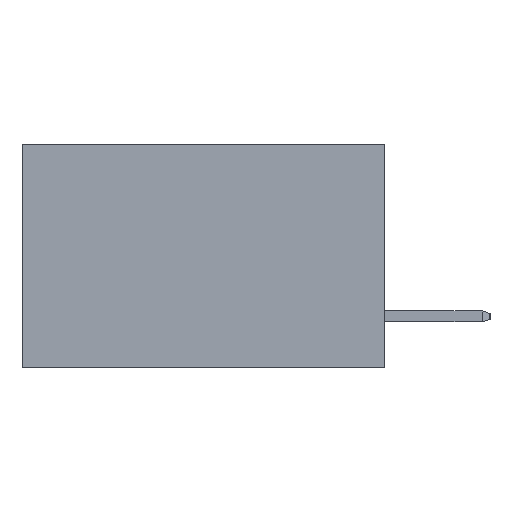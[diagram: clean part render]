
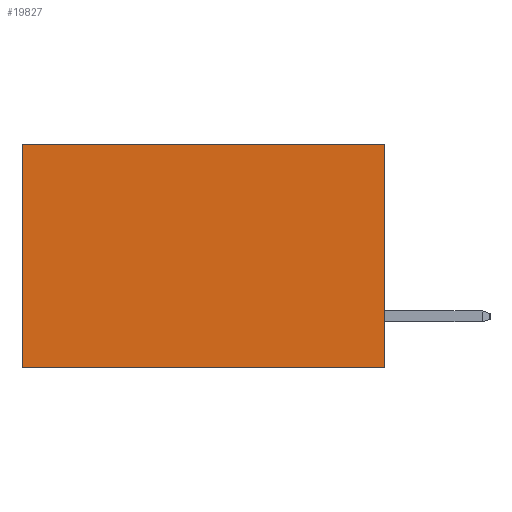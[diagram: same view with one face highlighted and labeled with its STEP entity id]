
A CAD part, left-side view. The second image highlights one B-rep face of the part: STEP entity #19827.
In plain terms, the highlighted planar face has unit normal (-1, 0, 0).
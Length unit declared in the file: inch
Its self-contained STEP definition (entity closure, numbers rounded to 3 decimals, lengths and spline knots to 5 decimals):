
#311 = DIRECTION ( 'NONE',  ( 0., 1., 0. ) ) ;
#355 = LINE ( 'NONE', #21070, #23672 ) ;
#1410 = DIRECTION ( 'NONE',  ( 0., 0., -1. ) ) ;
#2884 = CARTESIAN_POINT ( 'NONE',  ( 0.298, 0.6, 0. ) ) ;
#3209 = FACE_OUTER_BOUND ( 'NONE', #24162, .T. ) ;
#4001 = VERTEX_POINT ( 'NONE', #15580 ) ;
#4132 = ORIENTED_EDGE ( 'NONE', *, *, #22216, .F. ) ;
#4339 = LINE ( 'NONE', #30068, #28302 ) ;
#4352 = ORIENTED_EDGE ( 'NONE', *, *, #30662, .T. ) ;
#6212 = DIRECTION ( 'NONE',  ( 1., 0., 0. ) ) ;
#6879 = LINE ( 'NONE', #30172, #25953 ) ;
#8202 = CARTESIAN_POINT ( 'NONE',  ( 0.298, 0.6, -0.37 ) ) ;
#13429 = VECTOR ( 'NONE', #311, 39.37008 ) ;
#13577 = DIRECTION ( 'NONE',  ( 0., 0., -1. ) ) ;
#13687 = AXIS2_PLACEMENT_3D ( 'NONE', #20580, #6212, #22971 ) ;
#13732 = ORIENTED_EDGE ( 'NONE', *, *, #15930, .T. ) ;
#14002 = DIRECTION ( 'NONE',  ( 0., 1., 0. ) ) ;
#15580 = CARTESIAN_POINT ( 'NONE',  ( 0.298, 0., 0. ) ) ;
#15930 = EDGE_CURVE ( 'NONE', #25915, #20341, #6879, .T. ) ;
#17226 = VERTEX_POINT ( 'NONE', #24943 ) ;
#19485 = CARTESIAN_POINT ( 'NONE',  ( 0.298, 0., 0. ) ) ;
#19759 = LINE ( 'NONE', #19485, #13429 ) ;
#19827 = ADVANCED_FACE ( 'NONE', ( #3209 ), #25247, .F. ) ;
#20341 = VERTEX_POINT ( 'NONE', #8202 ) ;
#20580 = CARTESIAN_POINT ( 'NONE',  ( 0.298, 0., 0. ) ) ;
#21070 = CARTESIAN_POINT ( 'NONE',  ( 0.298, 0., -0.37 ) ) ;
#21430 = ORIENTED_EDGE ( 'NONE', *, *, #27681, .F. ) ;
#22216 = EDGE_CURVE ( 'NONE', #4001, #17226, #4339, .T. ) ;
#22971 = DIRECTION ( 'NONE',  ( 0., 0., -1. ) ) ;
#23672 = VECTOR ( 'NONE', #14002, 39.37008 ) ;
#24162 = EDGE_LOOP ( 'NONE', ( #13732, #21430, #4132, #4352 ) ) ;
#24943 = CARTESIAN_POINT ( 'NONE',  ( 0.298, 0., -0.37 ) ) ;
#25247 = PLANE ( 'NONE',  #13687 ) ;
#25915 = VERTEX_POINT ( 'NONE', #2884 ) ;
#25953 = VECTOR ( 'NONE', #13577, 39.37008 ) ;
#27681 = EDGE_CURVE ( 'NONE', #17226, #20341, #355, .T. ) ;
#28302 = VECTOR ( 'NONE', #1410, 39.37008 ) ;
#30068 = CARTESIAN_POINT ( 'NONE',  ( 0.298, 0., 0. ) ) ;
#30172 = CARTESIAN_POINT ( 'NONE',  ( 0.298, 0.6, 0. ) ) ;
#30662 = EDGE_CURVE ( 'NONE', #4001, #25915, #19759, .T. ) ;
